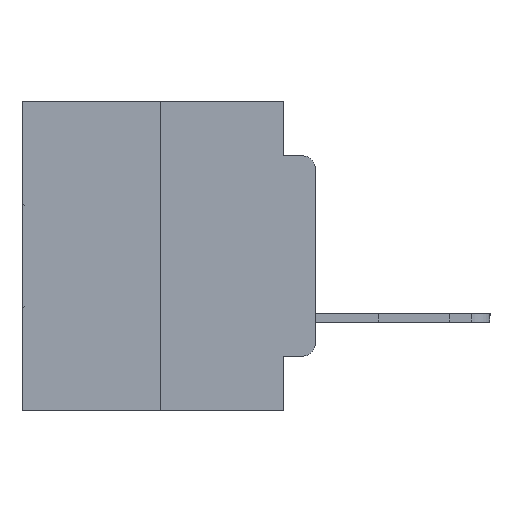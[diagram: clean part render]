
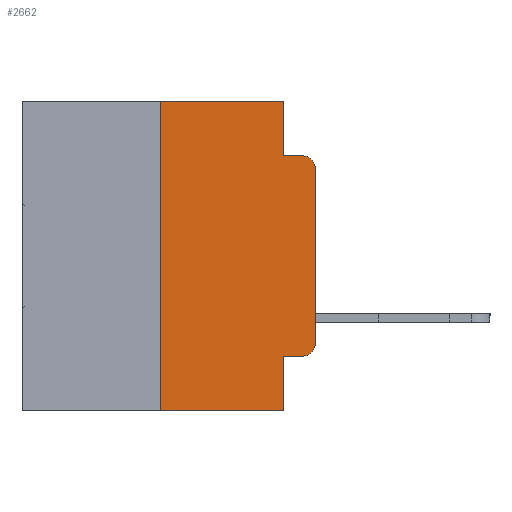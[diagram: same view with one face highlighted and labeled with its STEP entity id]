
A CAD part, left-side view. The second image highlights one B-rep face of the part: STEP entity #2662.
In plain terms, the highlighted planar face has unit normal (-1, 0, 0).
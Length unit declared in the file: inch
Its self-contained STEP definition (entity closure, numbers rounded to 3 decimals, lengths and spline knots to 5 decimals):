
#189 = AXIS2_PLACEMENT_3D ( 'NONE', #27095, #13712, #29295 ) ;
#893 = CARTESIAN_POINT ( 'NONE',  ( 0., 0., -0.3915 ) ) ;
#1223 = ORIENTED_EDGE ( 'NONE', *, *, #3988, .T. ) ;
#2478 = LINE ( 'NONE', #21105, #25924 ) ;
#2606 = CARTESIAN_POINT ( 'NONE',  ( 0., 0.02, -0.0885 ) ) ;
#2662 = ADVANCED_FACE ( 'NONE', ( #19445 ), #13525, .F. ) ;
#2954 = VECTOR ( 'NONE', #8378, 39.37008 ) ;
#3984 = VERTEX_POINT ( 'NONE', #12973 ) ;
#3988 = EDGE_CURVE ( 'NONE', #17127, #13644, #21146, .T. ) ;
#4354 = EDGE_LOOP ( 'NONE', ( #20938, #20608, #21064, #12682, #6570, #4454, #11381, #5741, #1223, #18287 ) ) ;
#4454 = ORIENTED_EDGE ( 'NONE', *, *, #28058, .F. ) ;
#4834 = VECTOR ( 'NONE', #26908, 39.37008 ) ;
#5206 = DIRECTION ( 'NONE',  ( 0., -1., 0. ) ) ;
#5267 = DIRECTION ( 'NONE',  ( 0., 0., -1. ) ) ;
#5741 = ORIENTED_EDGE ( 'NONE', *, *, #15351, .F. ) ;
#6570 = ORIENTED_EDGE ( 'NONE', *, *, #29086, .F. ) ;
#7429 = CIRCLE ( 'NONE', #9822, 0.02 ) ;
#7517 = CARTESIAN_POINT ( 'NONE',  ( 0., 0.473, 0. ) ) ;
#7802 = DIRECTION ( 'NONE',  ( 0., 0., 1. ) ) ;
#7937 = VECTOR ( 'NONE', #12198, 39.37008 ) ;
#8310 = VERTEX_POINT ( 'NONE', #24232 ) ;
#8378 = DIRECTION ( 'NONE',  ( 0., -1., 0. ) ) ;
#8451 = CARTESIAN_POINT ( 'NONE',  ( 0., 0.02, -0.1085 ) ) ;
#8701 = VERTEX_POINT ( 'NONE', #893 ) ;
#9822 = AXIS2_PLACEMENT_3D ( 'NONE', #8451, #24225, #10754 ) ;
#10679 = CARTESIAN_POINT ( 'NONE',  ( 0., 0.051, -0.4115 ) ) ;
#10681 = CARTESIAN_POINT ( 'NONE',  ( 0., 0.473, 0. ) ) ;
#10754 = DIRECTION ( 'NONE',  ( 0., 0., -1. ) ) ;
#10946 = EDGE_CURVE ( 'NONE', #8701, #24499, #17007, .T. ) ;
#11178 = CARTESIAN_POINT ( 'NONE',  ( 0., 0.051, -0.0885 ) ) ;
#11381 = ORIENTED_EDGE ( 'NONE', *, *, #18494, .T. ) ;
#11545 = VERTEX_POINT ( 'NONE', #20476 ) ;
#12198 = DIRECTION ( 'NONE',  ( 0., -1., 0. ) ) ;
#12682 = ORIENTED_EDGE ( 'NONE', *, *, #22457, .F. ) ;
#12843 = VERTEX_POINT ( 'NONE', #11178 ) ;
#12973 = CARTESIAN_POINT ( 'NONE',  ( 0., 0.051, -0.5 ) ) ;
#13114 = CARTESIAN_POINT ( 'NONE',  ( 0., 0.25, 0. ) ) ;
#13215 = VECTOR ( 'NONE', #24059, 39.37008 ) ;
#13266 = DIRECTION ( 'NONE',  ( 0., 0., -1. ) ) ;
#13353 = DIRECTION ( 'NONE',  ( 1., 0., 0. ) ) ;
#13525 = PLANE ( 'NONE',  #27816 ) ;
#13644 = VERTEX_POINT ( 'NONE', #25752 ) ;
#13712 = DIRECTION ( 'NONE',  ( -1., 0., 0. ) ) ;
#14916 = LINE ( 'NONE', #25453, #20199 ) ;
#14938 = EDGE_CURVE ( 'NONE', #24499, #19532, #7429, .T. ) ;
#15351 = EDGE_CURVE ( 'NONE', #17127, #3984, #14916, .T. ) ;
#15422 = LINE ( 'NONE', #23374, #7937 ) ;
#15471 = LINE ( 'NONE', #19119, #25978 ) ;
#17007 = LINE ( 'NONE', #24578, #4834 ) ;
#17127 = VERTEX_POINT ( 'NONE', #25650 ) ;
#18287 = ORIENTED_EDGE ( 'NONE', *, *, #21442, .T. ) ;
#18494 = EDGE_CURVE ( 'NONE', #8310, #3984, #2478, .T. ) ;
#18504 = EDGE_CURVE ( 'NONE', #12843, #19532, #15422, .T. ) ;
#18902 = CIRCLE ( 'NONE', #189, 0.02 ) ;
#19119 = CARTESIAN_POINT ( 'NONE',  ( 0., 0.25, 0. ) ) ;
#19445 = FACE_OUTER_BOUND ( 'NONE', #4354, .T. ) ;
#19532 = VERTEX_POINT ( 'NONE', #2606 ) ;
#20199 = VECTOR ( 'NONE', #5267, 39.37008 ) ;
#20476 = CARTESIAN_POINT ( 'NONE',  ( 0., 0.051, 0. ) ) ;
#20608 = ORIENTED_EDGE ( 'NONE', *, *, #14938, .T. ) ;
#20938 = ORIENTED_EDGE ( 'NONE', *, *, #10946, .T. ) ;
#21064 = ORIENTED_EDGE ( 'NONE', *, *, #18504, .F. ) ;
#21105 = CARTESIAN_POINT ( 'NONE',  ( 0., 0.473, -0.5 ) ) ;
#21146 = LINE ( 'NONE', #10679, #2954 ) ;
#21442 = EDGE_CURVE ( 'NONE', #13644, #8701, #18902, .T. ) ;
#21785 = CARTESIAN_POINT ( 'NONE',  ( 0., 0.051, 0. ) ) ;
#22457 = EDGE_CURVE ( 'NONE', #11545, #12843, #25117, .T. ) ;
#23374 = CARTESIAN_POINT ( 'NONE',  ( 0., 0.051, -0.0885 ) ) ;
#24059 = DIRECTION ( 'NONE',  ( 0., 0., -1. ) ) ;
#24143 = CARTESIAN_POINT ( 'NONE',  ( 0., 0., -0.1085 ) ) ;
#24225 = DIRECTION ( 'NONE',  ( -1., 0., 0. ) ) ;
#24232 = CARTESIAN_POINT ( 'NONE',  ( 0., 0.25, -0.5 ) ) ;
#24499 = VERTEX_POINT ( 'NONE', #24143 ) ;
#24578 = CARTESIAN_POINT ( 'NONE',  ( 0., 0., 0. ) ) ;
#25117 = LINE ( 'NONE', #21785, #13215 ) ;
#25453 = CARTESIAN_POINT ( 'NONE',  ( 0., 0.051, 0. ) ) ;
#25650 = CARTESIAN_POINT ( 'NONE',  ( 0., 0.051, -0.4115 ) ) ;
#25752 = CARTESIAN_POINT ( 'NONE',  ( 0., 0.02, -0.4115 ) ) ;
#25924 = VECTOR ( 'NONE', #5206, 39.37008 ) ;
#25978 = VECTOR ( 'NONE', #7802, 39.37008 ) ;
#26242 = LINE ( 'NONE', #10681, #26938 ) ;
#26365 = DIRECTION ( 'NONE',  ( 0., -1., 0. ) ) ;
#26908 = DIRECTION ( 'NONE',  ( 0., 0., 1. ) ) ;
#26938 = VECTOR ( 'NONE', #26365, 39.37008 ) ;
#27095 = CARTESIAN_POINT ( 'NONE',  ( 0., 0.02, -0.3915 ) ) ;
#27816 = AXIS2_PLACEMENT_3D ( 'NONE', #7517, #13353, #13266 ) ;
#28058 = EDGE_CURVE ( 'NONE', #8310, #28282, #15471, .T. ) ;
#28282 = VERTEX_POINT ( 'NONE', #13114 ) ;
#29086 = EDGE_CURVE ( 'NONE', #28282, #11545, #26242, .T. ) ;
#29295 = DIRECTION ( 'NONE',  ( 0., 0., -1. ) ) ;
